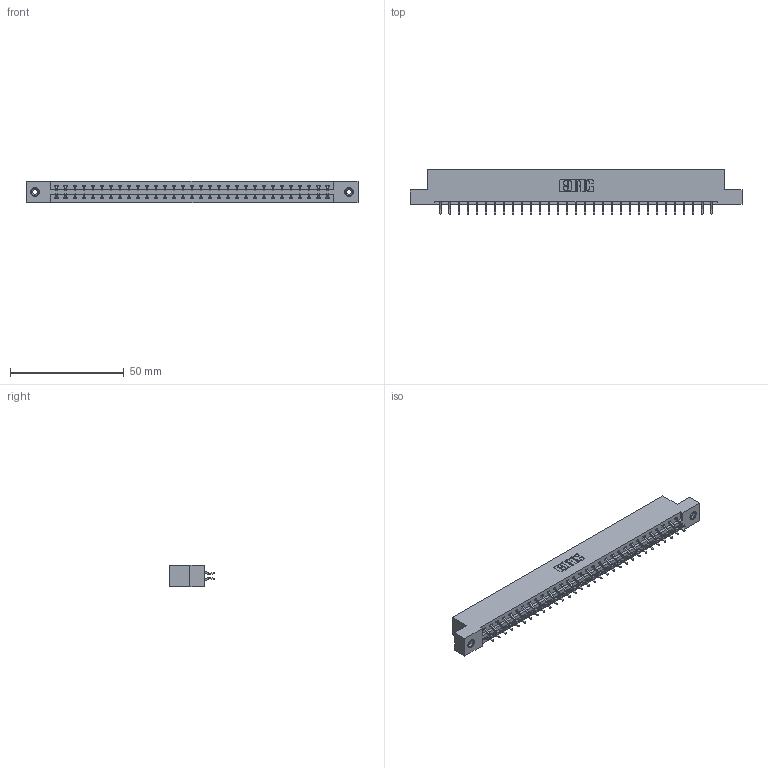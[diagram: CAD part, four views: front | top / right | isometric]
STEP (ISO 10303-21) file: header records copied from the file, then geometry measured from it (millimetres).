
FILE_DESCRIPTION (( 'STEP AP203' ), '1' );
FILE_NAME ('337-062-556-208.STEP', '2018-08-11T04:42:26', ( '' ), ( '' ), 'SwSTEP 2.0', 'SolidWorks 2016', '' );
FILE_SCHEMA (( 'CONFIG_CONTROL_DESIGN' ));
Length unit declared in the file: inch
Products named in the file (4): 345-250-001_345-250-003-102; 337-062-556-208; 337 Part_Flush Mounting Lugs - 0.156 Dia-TI; 345-292-001_556 Tail
Assembly tree (65 placements, depth 2):
  337-062-556-208
    337 Part_Flush Mounting Lugs - 0.156 Dia-TI
    345-292-001_556 Tail  x62
    345-250-001_345-250-003-102  x2
Bounding box: 145.85 x 19.57 x 9.4 mm (x, y, z)
Volume: 15215.1 mm3; surface area: 17052.4 mm2
Topology: 65 solids, 65 shells, 3894 faces, 11545 edges, 7606 vertices
Faces by surface type: plane 2706, cylinder 1172, cone 12, torus 4
Entity records: 26864 total; most frequent: CARTESIAN_POINT 4529, ORIENTED_EDGE 4446, DIRECTION 3893, EDGE_CURVE 2223, VECTOR 2067, LINE 2067, VERTEX_POINT 1476, AXIS2_PLACEMENT_3D 913
